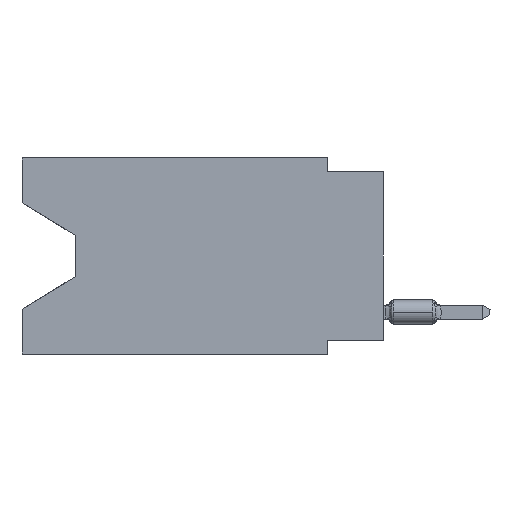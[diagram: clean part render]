
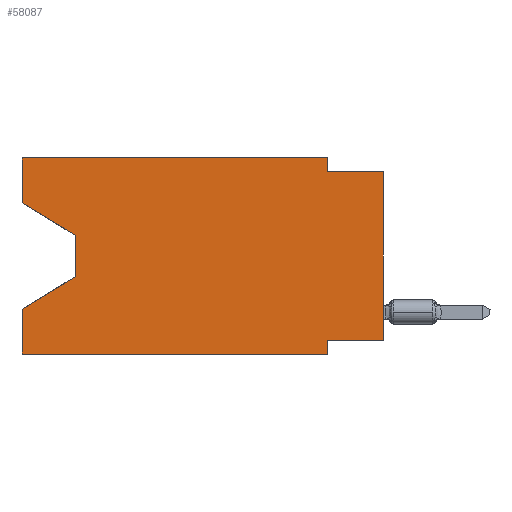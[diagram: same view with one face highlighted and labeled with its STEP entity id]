
A CAD part, left-side view. The second image highlights one B-rep face of the part: STEP entity #58087.
In plain terms, the highlighted planar face has unit normal (-1, 0, 0).
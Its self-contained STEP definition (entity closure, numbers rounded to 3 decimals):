
#15 = VERTEX_POINT ( 'NONE', #16340 ) ;
#1890 = VERTEX_POINT ( 'NONE', #34142 ) ;
#2367 = VERTEX_POINT ( 'NONE', #26794 ) ;
#2535 = CARTESIAN_POINT ( 'NONE',  ( 0., 0., -8.255 ) ) ;
#3589 = LINE ( 'NONE', #28065, #42094 ) ;
#3917 = DIRECTION ( 'NONE',  ( 0., 0., 1. ) ) ;
#4718 = VECTOR ( 'NONE', #17922, 1000. ) ;
#6595 = LINE ( 'NONE', #62034, #28532 ) ;
#6853 = VECTOR ( 'NONE', #42033, 1000. ) ;
#9165 = CARTESIAN_POINT ( 'NONE',  ( 0., 16.383, 0. ) ) ;
#9824 = VERTEX_POINT ( 'NONE', #19956 ) ;
#11523 = VERTEX_POINT ( 'NONE', #25356 ) ;
#11590 = EDGE_CURVE ( 'NONE', #36265, #63745, #34471, .T. ) ;
#12804 = EDGE_CURVE ( 'NONE', #32680, #15, #32621, .T. ) ;
#13243 = AXIS2_PLACEMENT_3D ( 'NONE', #14619, #54092, #14296 ) ;
#13887 = VECTOR ( 'NONE', #37504, 1000. ) ;
#14014 = EDGE_LOOP ( 'NONE', ( #38924, #15360, #19795, #28053, #17548, #42898, #59725, #24858, #42732, #52297, #36179, #33583 ) ) ;
#14090 = EDGE_CURVE ( 'NONE', #9824, #1890, #3589, .T. ) ;
#14296 = DIRECTION ( 'NONE',  ( 0., 0., -1. ) ) ;
#14327 = EDGE_CURVE ( 'NONE', #11523, #54717, #29666, .T. ) ;
#14619 = CARTESIAN_POINT ( 'NONE',  ( 0., 16.383, 0. ) ) ;
#14985 = CARTESIAN_POINT ( 'NONE',  ( 0., 2.54, -8.89 ) ) ;
#15360 = ORIENTED_EDGE ( 'NONE', *, *, #11590, .T. ) ;
#15939 = CARTESIAN_POINT ( 'NONE',  ( 0., 16.383, -2.038 ) ) ;
#16340 = CARTESIAN_POINT ( 'NONE',  ( 0., 16.383, 0. ) ) ;
#16849 = DIRECTION ( 'NONE',  ( 0., 0., -1. ) ) ;
#17266 = CARTESIAN_POINT ( 'NONE',  ( 0., 0., -0.635 ) ) ;
#17538 = DIRECTION ( 'NONE',  ( 0., 1., 0. ) ) ;
#17548 = ORIENTED_EDGE ( 'NONE', *, *, #14327, .T. ) ;
#17802 = EDGE_CURVE ( 'NONE', #32680, #36265, #22741, .T. ) ;
#17922 = DIRECTION ( 'NONE',  ( 0., -1., 0. ) ) ;
#18607 = DIRECTION ( 'NONE',  ( 0., 0., -1. ) ) ;
#19795 = ORIENTED_EDGE ( 'NONE', *, *, #55616, .T. ) ;
#19956 = CARTESIAN_POINT ( 'NONE',  ( 0., 0., -8.255 ) ) ;
#20531 = EDGE_CURVE ( 'NONE', #27097, #54717, #49229, .T. ) ;
#21145 = CARTESIAN_POINT ( 'NONE',  ( 0., 16.383, -6.852 ) ) ;
#22092 = DIRECTION ( 'NONE',  ( 0., -0.855, -0.519 ) ) ;
#22474 = CARTESIAN_POINT ( 'NONE',  ( 0., 13.97, -5.385 ) ) ;
#22741 = LINE ( 'NONE', #61271, #33961 ) ;
#23120 = FACE_OUTER_BOUND ( 'NONE', #14014, .T. ) ;
#24858 = ORIENTED_EDGE ( 'NONE', *, *, #14090, .T. ) ;
#25356 = CARTESIAN_POINT ( 'NONE',  ( 0., 16.383, -8.89 ) ) ;
#25430 = EDGE_CURVE ( 'NONE', #59199, #1890, #43017, .T. ) ;
#26794 = CARTESIAN_POINT ( 'NONE',  ( 0., 2.54, 0. ) ) ;
#27097 = VERTEX_POINT ( 'NONE', #46871 ) ;
#28053 = ORIENTED_EDGE ( 'NONE', *, *, #35299, .F. ) ;
#28065 = CARTESIAN_POINT ( 'NONE',  ( 0., 0., 0. ) ) ;
#28240 = VECTOR ( 'NONE', #16849, 1000. ) ;
#28479 = EDGE_CURVE ( 'NONE', #9824, #27097, #32214, .T. ) ;
#28532 = VECTOR ( 'NONE', #61715, 1000. ) ;
#29113 = VECTOR ( 'NONE', #37496, 1000. ) ;
#29594 = CARTESIAN_POINT ( 'NONE',  ( 0., 13.97, -3.505 ) ) ;
#29666 = LINE ( 'NONE', #49550, #44218 ) ;
#31322 = EDGE_CURVE ( 'NONE', #2367, #59199, #38141, .T. ) ;
#32214 = LINE ( 'NONE', #2535, #35201 ) ;
#32621 = LINE ( 'NONE', #51553, #13887 ) ;
#32680 = VERTEX_POINT ( 'NONE', #15939 ) ;
#33583 = ORIENTED_EDGE ( 'NONE', *, *, #12804, .F. ) ;
#33961 = VECTOR ( 'NONE', #22092, 1000. ) ;
#34142 = CARTESIAN_POINT ( 'NONE',  ( 0., 0., -0.635 ) ) ;
#34471 = LINE ( 'NONE', #29594, #28240 ) ;
#34572 = DIRECTION ( 'NONE',  ( 0., -1., 0. ) ) ;
#35201 = VECTOR ( 'NONE', #17538, 1000. ) ;
#35299 = EDGE_CURVE ( 'NONE', #11523, #64272, #6595, .T. ) ;
#36179 = ORIENTED_EDGE ( 'NONE', *, *, #42794, .F. ) ;
#36265 = VERTEX_POINT ( 'NONE', #60396 ) ;
#37174 = CARTESIAN_POINT ( 'NONE',  ( 0., 2.54, 0. ) ) ;
#37496 = DIRECTION ( 'NONE',  ( 0., 0., -1. ) ) ;
#37504 = DIRECTION ( 'NONE',  ( 0., 0., 1. ) ) ;
#38141 = LINE ( 'NONE', #37174, #29113 ) ;
#38924 = ORIENTED_EDGE ( 'NONE', *, *, #17802, .T. ) ;
#41522 = VECTOR ( 'NONE', #18607, 1000. ) ;
#42033 = DIRECTION ( 'NONE',  ( 0., 0.855, -0.519 ) ) ;
#42094 = VECTOR ( 'NONE', #3917, 1000. ) ;
#42732 = ORIENTED_EDGE ( 'NONE', *, *, #25430, .F. ) ;
#42794 = EDGE_CURVE ( 'NONE', #15, #2367, #59712, .T. ) ;
#42898 = ORIENTED_EDGE ( 'NONE', *, *, #20531, .F. ) ;
#43017 = LINE ( 'NONE', #17266, #4718 ) ;
#44218 = VECTOR ( 'NONE', #46924, 1000. ) ;
#44443 = CARTESIAN_POINT ( 'NONE',  ( 0., 2.54, -0.635 ) ) ;
#46871 = CARTESIAN_POINT ( 'NONE',  ( 0., 2.54, -8.255 ) ) ;
#46924 = DIRECTION ( 'NONE',  ( 0., -1., 0. ) ) ;
#48546 = PLANE ( 'NONE',  #13243 ) ;
#49229 = LINE ( 'NONE', #14985, #41522 ) ;
#49550 = CARTESIAN_POINT ( 'NONE',  ( 0., 16.383, -8.89 ) ) ;
#51553 = CARTESIAN_POINT ( 'NONE',  ( 0., 16.383, 0. ) ) ;
#52297 = ORIENTED_EDGE ( 'NONE', *, *, #31322, .F. ) ;
#53938 = CARTESIAN_POINT ( 'NONE',  ( 0., 13.97, -5.385 ) ) ;
#54092 = DIRECTION ( 'NONE',  ( 1., 0., 0. ) ) ;
#54717 = VERTEX_POINT ( 'NONE', #62943 ) ;
#55616 = EDGE_CURVE ( 'NONE', #63745, #64272, #62612, .T. ) ;
#58087 = ADVANCED_FACE ( 'NONE', ( #23120 ), #48546, .F. ) ;
#58402 = VECTOR ( 'NONE', #34572, 1000. ) ;
#59199 = VERTEX_POINT ( 'NONE', #44443 ) ;
#59712 = LINE ( 'NONE', #9165, #58402 ) ;
#59725 = ORIENTED_EDGE ( 'NONE', *, *, #28479, .F. ) ;
#60396 = CARTESIAN_POINT ( 'NONE',  ( 0., 13.97, -3.505 ) ) ;
#61271 = CARTESIAN_POINT ( 'NONE',  ( 0., 16.383, -2.038 ) ) ;
#61715 = DIRECTION ( 'NONE',  ( 0., 0., 1. ) ) ;
#62034 = CARTESIAN_POINT ( 'NONE',  ( 0., 16.383, 0. ) ) ;
#62612 = LINE ( 'NONE', #22474, #6853 ) ;
#62943 = CARTESIAN_POINT ( 'NONE',  ( 0., 2.54, -8.89 ) ) ;
#63745 = VERTEX_POINT ( 'NONE', #53938 ) ;
#64272 = VERTEX_POINT ( 'NONE', #21145 ) ;
